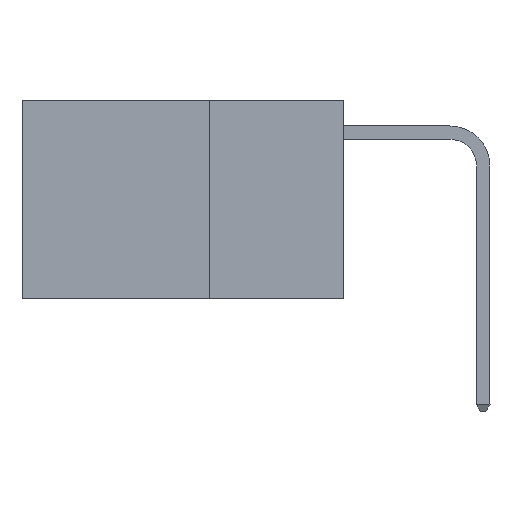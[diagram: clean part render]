
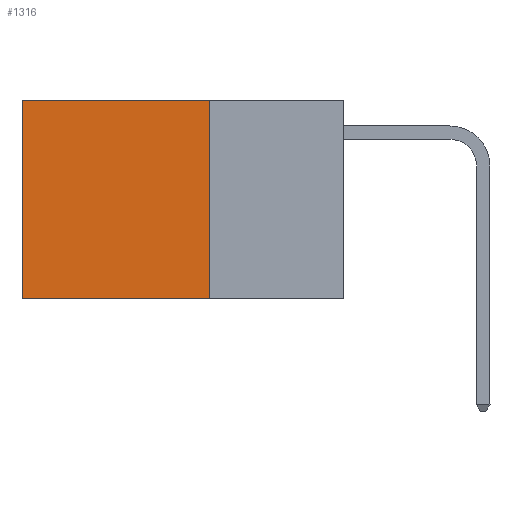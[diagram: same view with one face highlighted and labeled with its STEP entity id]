
A CAD part, left-side view. The second image highlights one B-rep face of the part: STEP entity #1316.
In plain terms, the highlighted planar face has unit normal (-1, 0, 0).
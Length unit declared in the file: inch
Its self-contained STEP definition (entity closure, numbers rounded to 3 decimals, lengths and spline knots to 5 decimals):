
#206 = VERTEX_POINT ( 'NONE', #1098 ) ;
#273 = VECTOR ( 'NONE', #7010, 39.37008 ) ;
#425 = EDGE_LOOP ( 'NONE', ( #12197, #7273, #12088, #15376 ) ) ;
#457 = DIRECTION ( 'NONE',  ( 0., 0., -1. ) ) ;
#1098 = CARTESIAN_POINT ( 'NONE',  ( 0.2625, 0.6, 0. ) ) ;
#1279 = DIRECTION ( 'NONE',  ( 0., 1., 0. ) ) ;
#1316 = ADVANCED_FACE ( 'NONE', ( #1935 ), #2426, .F. ) ;
#1935 = FACE_OUTER_BOUND ( 'NONE', #425, .T. ) ;
#2136 = LINE ( 'NONE', #16442, #10800 ) ;
#2154 = CARTESIAN_POINT ( 'NONE',  ( 0.2625, 0.25, 0. ) ) ;
#2224 = VECTOR ( 'NONE', #1279, 39.37008 ) ;
#2426 = PLANE ( 'NONE',  #8780 ) ;
#3629 = DIRECTION ( 'NONE',  ( 1., 0., 0. ) ) ;
#3747 = VERTEX_POINT ( 'NONE', #7132 ) ;
#3884 = VERTEX_POINT ( 'NONE', #7307 ) ;
#5097 = CARTESIAN_POINT ( 'NONE',  ( 0.2625, 0.25, 0. ) ) ;
#7010 = DIRECTION ( 'NONE',  ( 0., 0., -1. ) ) ;
#7132 = CARTESIAN_POINT ( 'NONE',  ( 0.2625, 0.25, -0.37 ) ) ;
#7273 = ORIENTED_EDGE ( 'NONE', *, *, #9785, .F. ) ;
#7307 = CARTESIAN_POINT ( 'NONE',  ( 0.2625, 0.6, -0.37 ) ) ;
#7429 = LINE ( 'NONE', #2154, #273 ) ;
#7697 = CARTESIAN_POINT ( 'NONE',  ( 0.2625, 0.25, 0. ) ) ;
#7849 = LINE ( 'NONE', #5097, #2224 ) ;
#8780 = AXIS2_PLACEMENT_3D ( 'NONE', #7697, #3629, #457 ) ;
#8823 = CARTESIAN_POINT ( 'NONE',  ( 0.2625, 0.25, 0. ) ) ;
#9785 = EDGE_CURVE ( 'NONE', #3747, #3884, #10060, .T. ) ;
#10060 = LINE ( 'NONE', #11374, #15772 ) ;
#10412 = EDGE_CURVE ( 'NONE', #12894, #206, #7849, .T. ) ;
#10800 = VECTOR ( 'NONE', #15457, 39.37008 ) ;
#11374 = CARTESIAN_POINT ( 'NONE',  ( 0.2625, 0.25, -0.37 ) ) ;
#11906 = EDGE_CURVE ( 'NONE', #12894, #3747, #7429, .T. ) ;
#12088 = ORIENTED_EDGE ( 'NONE', *, *, #11906, .F. ) ;
#12197 = ORIENTED_EDGE ( 'NONE', *, *, #12351, .T. ) ;
#12351 = EDGE_CURVE ( 'NONE', #206, #3884, #2136, .T. ) ;
#12894 = VERTEX_POINT ( 'NONE', #8823 ) ;
#15376 = ORIENTED_EDGE ( 'NONE', *, *, #10412, .T. ) ;
#15377 = DIRECTION ( 'NONE',  ( 0., 1., 0. ) ) ;
#15457 = DIRECTION ( 'NONE',  ( 0., 0., -1. ) ) ;
#15772 = VECTOR ( 'NONE', #15377, 39.37008 ) ;
#16442 = CARTESIAN_POINT ( 'NONE',  ( 0.2625, 0.6, 0. ) ) ;
